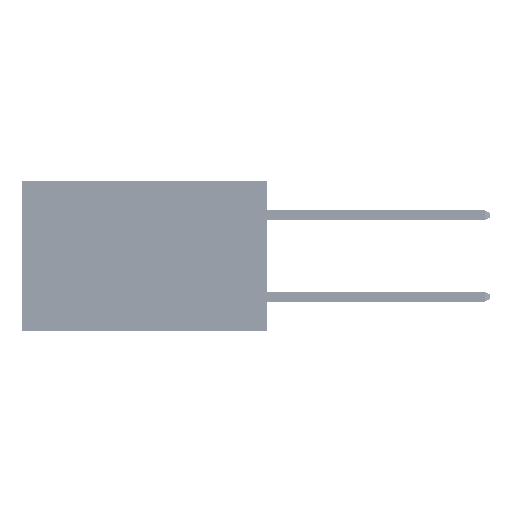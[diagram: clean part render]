
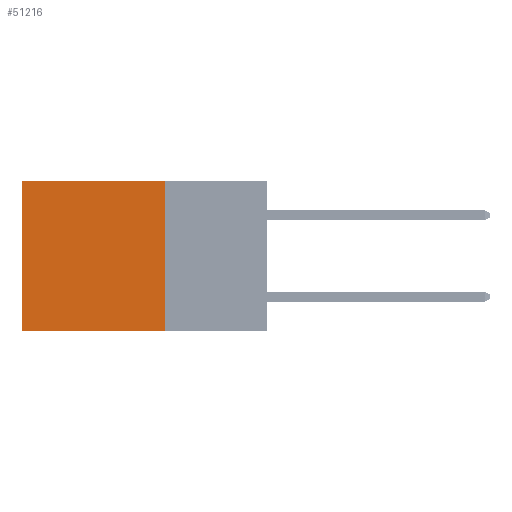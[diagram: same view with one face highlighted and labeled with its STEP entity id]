
A CAD part, left-side view. The second image highlights one B-rep face of the part: STEP entity #51216.
In plain terms, the highlighted planar face has unit normal (-1, 0, 0).
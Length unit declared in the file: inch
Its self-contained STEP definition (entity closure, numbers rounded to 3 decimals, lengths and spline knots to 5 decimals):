
#1139 = CARTESIAN_POINT ( 'NONE',  ( 0.2875, 0.25, 0. ) ) ;
#2376 = ORIENTED_EDGE ( 'NONE', *, *, #22010, .F. ) ;
#3141 = VECTOR ( 'NONE', #18242, 39.37008 ) ;
#3156 = DIRECTION ( 'NONE',  ( 0., 0., -1. ) ) ;
#3633 = ORIENTED_EDGE ( 'NONE', *, *, #33902, .F. ) ;
#5074 = ORIENTED_EDGE ( 'NONE', *, *, #41605, .T. ) ;
#5224 = EDGE_LOOP ( 'NONE', ( #48106, #3633, #2376, #5074 ) ) ;
#6664 = CARTESIAN_POINT ( 'NONE',  ( 0.2875, 0.25, -0.37 ) ) ;
#6816 = AXIS2_PLACEMENT_3D ( 'NONE', #7718, #23865, #8063 ) ;
#7718 = CARTESIAN_POINT ( 'NONE',  ( 0.2875, 0.25, 0. ) ) ;
#8063 = DIRECTION ( 'NONE',  ( 0., 0., -1. ) ) ;
#9385 = LINE ( 'NONE', #23463, #43886 ) ;
#10225 = CARTESIAN_POINT ( 'NONE',  ( 0.2875, 0.25, 0. ) ) ;
#14668 = CARTESIAN_POINT ( 'NONE',  ( 0.2875, 0.6, 0. ) ) ;
#15664 = LINE ( 'NONE', #6664, #3141 ) ;
#17231 = DIRECTION ( 'NONE',  ( 0., 1., 0. ) ) ;
#18242 = DIRECTION ( 'NONE',  ( 0., 1., 0. ) ) ;
#21982 = FACE_OUTER_BOUND ( 'NONE', #5224, .T. ) ;
#22010 = EDGE_CURVE ( 'NONE', #30750, #46849, #9385, .T. ) ;
#23463 = CARTESIAN_POINT ( 'NONE',  ( 0.2875, 0.25, 0. ) ) ;
#23865 = DIRECTION ( 'NONE',  ( 1., 0., 0. ) ) ;
#27218 = EDGE_CURVE ( 'NONE', #33122, #47244, #36740, .T. ) ;
#27728 = PLANE ( 'NONE',  #6816 ) ;
#27911 = CARTESIAN_POINT ( 'NONE',  ( 0.2875, 0.6, -0.37 ) ) ;
#30750 = VERTEX_POINT ( 'NONE', #10225 ) ;
#33122 = VERTEX_POINT ( 'NONE', #45644 ) ;
#33648 = VECTOR ( 'NONE', #17231, 39.37008 ) ;
#33902 = EDGE_CURVE ( 'NONE', #46849, #47244, #15664, .T. ) ;
#33933 = DIRECTION ( 'NONE',  ( 0., 0., -1. ) ) ;
#36740 = LINE ( 'NONE', #14668, #40560 ) ;
#38088 = CARTESIAN_POINT ( 'NONE',  ( 0.2875, 0.25, -0.37 ) ) ;
#40560 = VECTOR ( 'NONE', #33933, 39.37008 ) ;
#41605 = EDGE_CURVE ( 'NONE', #30750, #33122, #43654, .T. ) ;
#43654 = LINE ( 'NONE', #1139, #33648 ) ;
#43886 = VECTOR ( 'NONE', #3156, 39.37008 ) ;
#45644 = CARTESIAN_POINT ( 'NONE',  ( 0.2875, 0.6, 0. ) ) ;
#46849 = VERTEX_POINT ( 'NONE', #38088 ) ;
#47244 = VERTEX_POINT ( 'NONE', #27911 ) ;
#48106 = ORIENTED_EDGE ( 'NONE', *, *, #27218, .T. ) ;
#51216 = ADVANCED_FACE ( 'NONE', ( #21982 ), #27728, .F. ) ;
